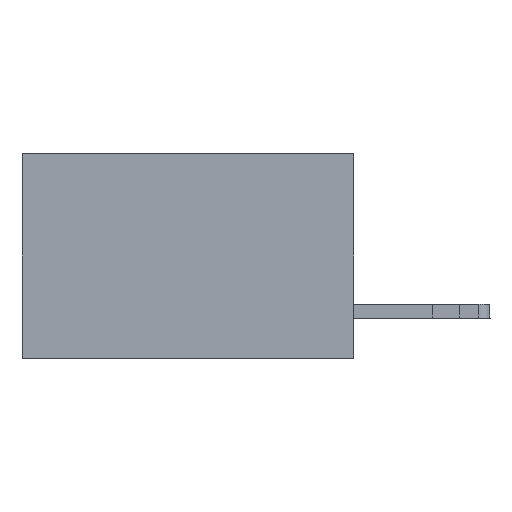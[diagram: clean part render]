
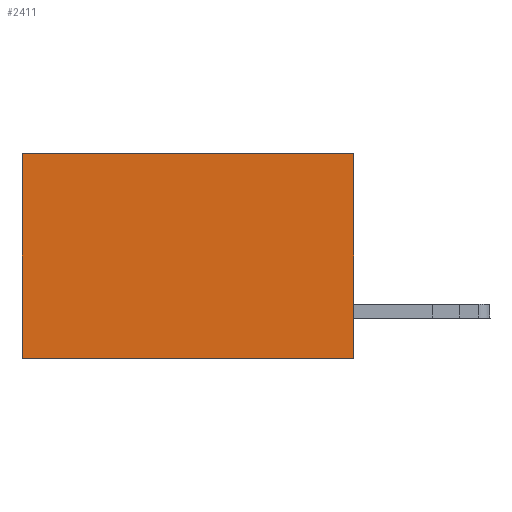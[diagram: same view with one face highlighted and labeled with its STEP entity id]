
A CAD part, left-side view. The second image highlights one B-rep face of the part: STEP entity #2411.
In plain terms, the highlighted planar face has unit normal (-1, 0, 0).
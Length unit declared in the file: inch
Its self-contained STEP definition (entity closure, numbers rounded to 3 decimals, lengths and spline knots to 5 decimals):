
#912 = ORIENTED_EDGE ( 'NONE', *, *, #2134, .T. ) ;
#1648 = DIRECTION ( 'NONE',  ( 0., 0., -1. ) ) ;
#1836 = CARTESIAN_POINT ( 'NONE',  ( 0.2875, 0.6, 0. ) ) ;
#2134 = EDGE_CURVE ( 'NONE', #5551, #3621, #10580, .T. ) ;
#2411 = ADVANCED_FACE ( 'NONE', ( #12685 ), #14878, .F. ) ;
#2983 = ORIENTED_EDGE ( 'NONE', *, *, #3901, .F. ) ;
#3386 = DIRECTION ( 'NONE',  ( 0., 1., 0. ) ) ;
#3410 = CARTESIAN_POINT ( 'NONE',  ( 0.2875, 0., 0. ) ) ;
#3501 = VECTOR ( 'NONE', #15446, 39.37008 ) ;
#3606 = ORIENTED_EDGE ( 'NONE', *, *, #16707, .F. ) ;
#3621 = VERTEX_POINT ( 'NONE', #10714 ) ;
#3901 = EDGE_CURVE ( 'NONE', #10290, #3621, #12840, .T. ) ;
#4149 = DIRECTION ( 'NONE',  ( 0., 0., -1. ) ) ;
#5474 = DIRECTION ( 'NONE',  ( 1., 0., 0. ) ) ;
#5551 = VERTEX_POINT ( 'NONE', #8047 ) ;
#6696 = VERTEX_POINT ( 'NONE', #3410 ) ;
#7005 = CARTESIAN_POINT ( 'NONE',  ( 0.2875, 0., -0.37 ) ) ;
#7107 = AXIS2_PLACEMENT_3D ( 'NONE', #17136, #5474, #4149 ) ;
#7380 = VECTOR ( 'NONE', #1648, 39.37008 ) ;
#8047 = CARTESIAN_POINT ( 'NONE',  ( 0.2875, 0.6, 0. ) ) ;
#8726 = ORIENTED_EDGE ( 'NONE', *, *, #9426, .T. ) ;
#9291 = VECTOR ( 'NONE', #14713, 39.37008 ) ;
#9310 = CARTESIAN_POINT ( 'NONE',  ( 0.2875, 0., 0. ) ) ;
#9426 = EDGE_CURVE ( 'NONE', #6696, #5551, #9691, .T. ) ;
#9691 = LINE ( 'NONE', #9310, #9291 ) ;
#10290 = VERTEX_POINT ( 'NONE', #7005 ) ;
#10580 = LINE ( 'NONE', #1836, #7380 ) ;
#10714 = CARTESIAN_POINT ( 'NONE',  ( 0.2875, 0.6, -0.37 ) ) ;
#12415 = VECTOR ( 'NONE', #3386, 39.37008 ) ;
#12685 = FACE_OUTER_BOUND ( 'NONE', #16006, .T. ) ;
#12840 = LINE ( 'NONE', #16957, #12415 ) ;
#14172 = CARTESIAN_POINT ( 'NONE',  ( 0.2875, 0., 0. ) ) ;
#14713 = DIRECTION ( 'NONE',  ( 0., 1., 0. ) ) ;
#14878 = PLANE ( 'NONE',  #7107 ) ;
#15446 = DIRECTION ( 'NONE',  ( 0., 0., -1. ) ) ;
#16006 = EDGE_LOOP ( 'NONE', ( #912, #2983, #3606, #8726 ) ) ;
#16707 = EDGE_CURVE ( 'NONE', #6696, #10290, #17041, .T. ) ;
#16957 = CARTESIAN_POINT ( 'NONE',  ( 0.2875, 0., -0.37 ) ) ;
#17041 = LINE ( 'NONE', #14172, #3501 ) ;
#17136 = CARTESIAN_POINT ( 'NONE',  ( 0.2875, 0., 0. ) ) ;
